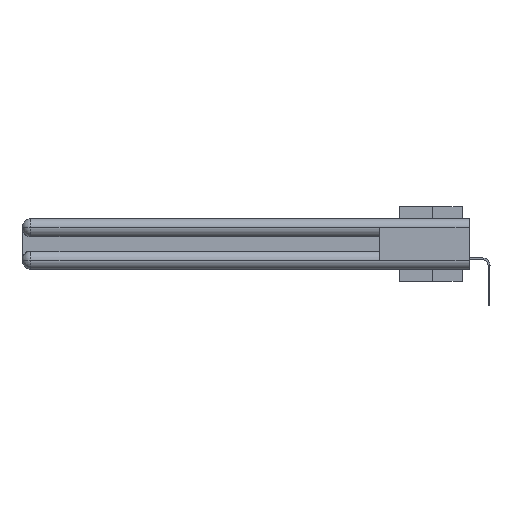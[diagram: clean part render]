
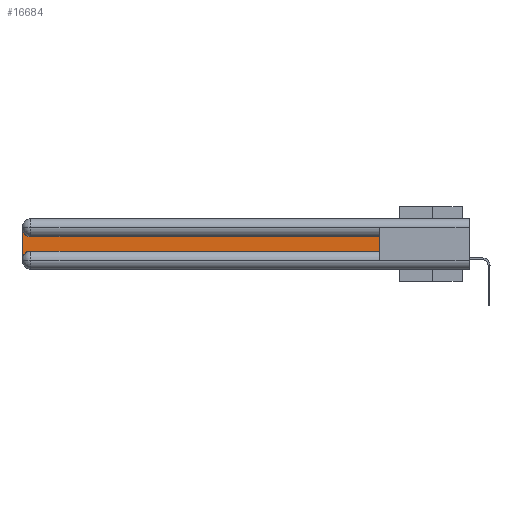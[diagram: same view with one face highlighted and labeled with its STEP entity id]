
A CAD part, left-side view. The second image highlights one B-rep face of the part: STEP entity #16684.
In plain terms, the highlighted planar face has unit normal (-1, 0, 0).
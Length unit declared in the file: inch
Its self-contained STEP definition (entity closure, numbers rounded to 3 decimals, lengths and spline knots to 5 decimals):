
#1100 = CARTESIAN_POINT ( 'NONE',  ( 0.075, 2.94, -0.0625 ) ) ;
#1428 = CARTESIAN_POINT ( 'NONE',  ( 0.075, 0.6, -0.2175 ) ) ;
#3498 = DIRECTION ( 'NONE',  ( 0., 0., -1. ) ) ;
#3660 = LINE ( 'NONE', #36050, #28378 ) ;
#3865 = CIRCLE ( 'NONE', #9857, 0.06 ) ;
#4291 = ORIENTED_EDGE ( 'NONE', *, *, #7206, .T. ) ;
#5486 = AXIS2_PLACEMENT_3D ( 'NONE', #12230, #28965, #20323 ) ;
#7134 = DIRECTION ( 'NONE',  ( 0., -1., 0. ) ) ;
#7206 = EDGE_CURVE ( 'NONE', #24330, #28428, #13835, .T. ) ;
#7283 = CARTESIAN_POINT ( 'NONE',  ( 0.075, 3., -0.2775 ) ) ;
#8394 = EDGE_CURVE ( 'NONE', #28428, #12009, #3865, .T. ) ;
#9389 = PLANE ( 'NONE',  #5486 ) ;
#9809 = ORIENTED_EDGE ( 'NONE', *, *, #10861, .T. ) ;
#9857 = AXIS2_PLACEMENT_3D ( 'NONE', #23342, #18006, #3498 ) ;
#10087 = CARTESIAN_POINT ( 'NONE',  ( 0.075, 0.6, -0.2175 ) ) ;
#10861 = EDGE_CURVE ( 'NONE', #11985, #30839, #3660, .T. ) ;
#11021 = AXIS2_PLACEMENT_3D ( 'NONE', #1100, #26862, #29690 ) ;
#11985 = VERTEX_POINT ( 'NONE', #27329 ) ;
#12009 = VERTEX_POINT ( 'NONE', #24735 ) ;
#12230 = CARTESIAN_POINT ( 'NONE',  ( 0.075, 3., -0.1225 ) ) ;
#13389 = DIRECTION ( 'NONE',  ( 0., 1., 0. ) ) ;
#13835 = LINE ( 'NONE', #31424, #27049 ) ;
#15034 = ORIENTED_EDGE ( 'NONE', *, *, #30863, .T. ) ;
#15203 = FACE_OUTER_BOUND ( 'NONE', #20834, .T. ) ;
#16684 = ADVANCED_FACE ( 'NONE', ( #15203 ), #9389, .F. ) ;
#17285 = VERTEX_POINT ( 'NONE', #10087 ) ;
#18006 = DIRECTION ( 'NONE',  ( 1., 0., 0. ) ) ;
#19761 = CARTESIAN_POINT ( 'NONE',  ( 0.075, 0.6, -0.2175 ) ) ;
#20323 = DIRECTION ( 'NONE',  ( 0., 0., -1. ) ) ;
#20511 = VECTOR ( 'NONE', #7134, 39.37008 ) ;
#20834 = EDGE_LOOP ( 'NONE', ( #9809, #23056, #4291, #26590, #15034, #22180 ) ) ;
#21636 = VECTOR ( 'NONE', #34221, 39.37008 ) ;
#22180 = ORIENTED_EDGE ( 'NONE', *, *, #27874, .T. ) ;
#23056 = ORIENTED_EDGE ( 'NONE', *, *, #30289, .T. ) ;
#23267 = DIRECTION ( 'NONE',  ( 0., 0., -1. ) ) ;
#23342 = CARTESIAN_POINT ( 'NONE',  ( 0.075, 2.94, -0.2775 ) ) ;
#23631 = LINE ( 'NONE', #1428, #20511 ) ;
#24330 = VERTEX_POINT ( 'NONE', #33048 ) ;
#24735 = CARTESIAN_POINT ( 'NONE',  ( 0.075, 2.94, -0.2175 ) ) ;
#26590 = ORIENTED_EDGE ( 'NONE', *, *, #8394, .T. ) ;
#26862 = DIRECTION ( 'NONE',  ( 1., 0., 0. ) ) ;
#27049 = VECTOR ( 'NONE', #23267, 39.37008 ) ;
#27329 = CARTESIAN_POINT ( 'NONE',  ( 0.075, 0.6, -0.1225 ) ) ;
#27874 = EDGE_CURVE ( 'NONE', #17285, #11985, #28278, .T. ) ;
#28278 = LINE ( 'NONE', #19761, #21636 ) ;
#28378 = VECTOR ( 'NONE', #13389, 39.37008 ) ;
#28428 = VERTEX_POINT ( 'NONE', #7283 ) ;
#28965 = DIRECTION ( 'NONE',  ( 1., 0., 0. ) ) ;
#29690 = DIRECTION ( 'NONE',  ( 0., 0., -1. ) ) ;
#30289 = EDGE_CURVE ( 'NONE', #30839, #24330, #35189, .T. ) ;
#30839 = VERTEX_POINT ( 'NONE', #32380 ) ;
#30863 = EDGE_CURVE ( 'NONE', #12009, #17285, #23631, .T. ) ;
#31424 = CARTESIAN_POINT ( 'NONE',  ( 0.075, 3., -0.2175 ) ) ;
#32380 = CARTESIAN_POINT ( 'NONE',  ( 0.075, 2.94, -0.1225 ) ) ;
#33048 = CARTESIAN_POINT ( 'NONE',  ( 0.075, 3., -0.0625 ) ) ;
#34221 = DIRECTION ( 'NONE',  ( 0., 0., 1. ) ) ;
#35189 = CIRCLE ( 'NONE', #11021, 0.06 ) ;
#36050 = CARTESIAN_POINT ( 'NONE',  ( 0.075, 0.6, -0.1225 ) ) ;
